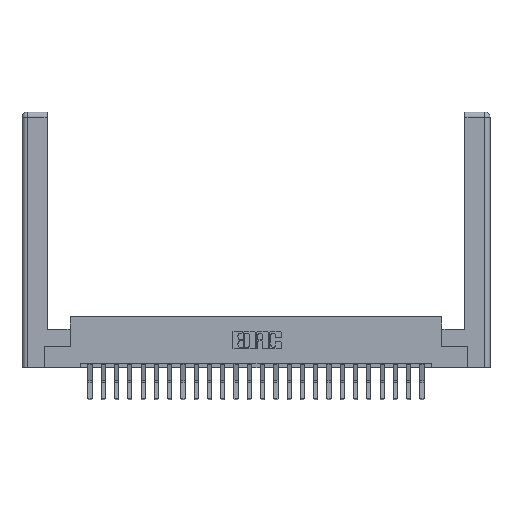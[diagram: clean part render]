
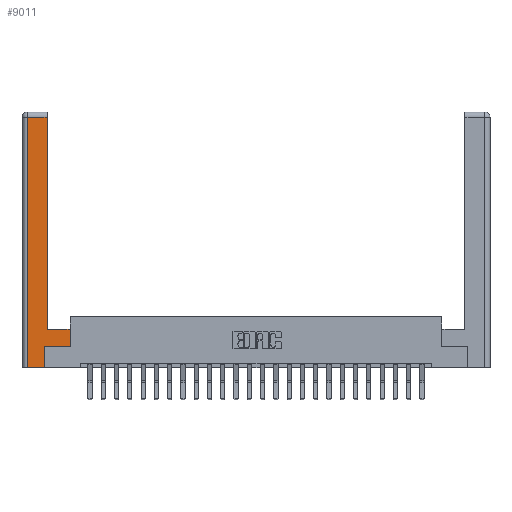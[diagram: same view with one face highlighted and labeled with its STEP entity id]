
A CAD part, top view. The second image highlights one B-rep face of the part: STEP entity #9011.
In plain terms, the highlighted planar face has unit normal (0, 0, 1).
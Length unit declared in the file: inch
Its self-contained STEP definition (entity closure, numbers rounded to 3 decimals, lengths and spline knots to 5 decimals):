
#345 = DIRECTION ( 'NONE',  ( 0., -1., 0. ) ) ;
#403 = FACE_OUTER_BOUND ( 'NONE', #6809, .T. ) ;
#785 = EDGE_CURVE ( 'NONE', #9974, #18784, #2170, .T. ) ;
#1206 = VECTOR ( 'NONE', #19770, 39.37008 ) ;
#2170 = LINE ( 'NONE', #8299, #19724 ) ;
#2855 = CARTESIAN_POINT ( 'NONE',  ( 0.295, 0.45, 0. ) ) ;
#3918 = ORIENTED_EDGE ( 'NONE', *, *, #5285, .T. ) ;
#4222 = ORIENTED_EDGE ( 'NONE', *, *, #16011, .T. ) ;
#4379 = CARTESIAN_POINT ( 'NONE',  ( 0.565, 0.45, 0. ) ) ;
#4415 = CARTESIAN_POINT ( 'NONE',  ( 0.265, 0.245, 0. ) ) ;
#4665 = VECTOR ( 'NONE', #4693, 39.37008 ) ;
#4693 = DIRECTION ( 'NONE',  ( 1., 0., 0. ) ) ;
#5285 = EDGE_CURVE ( 'NONE', #18784, #9771, #23835, .T. ) ;
#6759 = LINE ( 'NONE', #23803, #4665 ) ;
#6809 = EDGE_LOOP ( 'NONE', ( #21625, #19039, #19291, #3918, #19736, #19445, #9357, #4222 ) ) ;
#7153 = DIRECTION ( 'NONE',  ( 0., 0., -1. ) ) ;
#8011 = EDGE_CURVE ( 'NONE', #9771, #23929, #17389, .T. ) ;
#8299 = CARTESIAN_POINT ( 'NONE',  ( 0.0615, 0., 0. ) ) ;
#8806 = DIRECTION ( 'NONE',  ( -1., 0., 0. ) ) ;
#8950 = VECTOR ( 'NONE', #11927, 39.37008 ) ;
#8970 = VECTOR ( 'NONE', #15876, 39.37008 ) ;
#9011 = ADVANCED_FACE ( 'NONE', ( #403 ), #10373, .F. ) ;
#9092 = EDGE_CURVE ( 'NONE', #23929, #13352, #6759, .T. ) ;
#9189 = EDGE_CURVE ( 'NONE', #24588, #10053, #17122, .T. ) ;
#9357 = ORIENTED_EDGE ( 'NONE', *, *, #20486, .T. ) ;
#9771 = VERTEX_POINT ( 'NONE', #15657 ) ;
#9974 = VERTEX_POINT ( 'NONE', #13013 ) ;
#10053 = VERTEX_POINT ( 'NONE', #19138 ) ;
#10373 = PLANE ( 'NONE',  #14374 ) ;
#11901 = LINE ( 'NONE', #4379, #21228 ) ;
#11927 = DIRECTION ( 'NONE',  ( 0., 1., 0. ) ) ;
#11974 = CARTESIAN_POINT ( 'NONE',  ( 0.295, 3., 0. ) ) ;
#12408 = LINE ( 'NONE', #19405, #12727 ) ;
#12562 = CARTESIAN_POINT ( 'NONE',  ( 0., 0., 0. ) ) ;
#12727 = VECTOR ( 'NONE', #15801, 39.37008 ) ;
#12949 = CARTESIAN_POINT ( 'NONE',  ( 0.565, 0.245, 0. ) ) ;
#13013 = CARTESIAN_POINT ( 'NONE',  ( 0.0615, 2.94, 0. ) ) ;
#13352 = VERTEX_POINT ( 'NONE', #12949 ) ;
#13802 = CARTESIAN_POINT ( 'NONE',  ( 0.265, 0.245, 0. ) ) ;
#14374 = AXIS2_PLACEMENT_3D ( 'NONE', #12562, #7153, #14779 ) ;
#14396 = CARTESIAN_POINT ( 'NONE',  ( 0.565, 0.45, 0. ) ) ;
#14779 = DIRECTION ( 'NONE',  ( -1., 0., 0. ) ) ;
#14842 = CARTESIAN_POINT ( 'NONE',  ( 0.295, 0.45, 0. ) ) ;
#15657 = CARTESIAN_POINT ( 'NONE',  ( 0.265, 0., 0. ) ) ;
#15801 = DIRECTION ( 'NONE',  ( -1., 0., 0. ) ) ;
#15874 = CARTESIAN_POINT ( 'NONE',  ( 0.0615, 0., 0. ) ) ;
#15876 = DIRECTION ( 'NONE',  ( 0., 1., 0. ) ) ;
#16011 = EDGE_CURVE ( 'NONE', #19501, #24588, #24193, .T. ) ;
#16039 = DIRECTION ( 'NONE',  ( 0., 1., 0. ) ) ;
#16360 = EDGE_CURVE ( 'NONE', #10053, #9974, #12408, .T. ) ;
#16387 = VECTOR ( 'NONE', #8806, 39.37008 ) ;
#17122 = LINE ( 'NONE', #11974, #8970 ) ;
#17367 = CARTESIAN_POINT ( 'NONE',  ( 0.265, 0., 0. ) ) ;
#17389 = LINE ( 'NONE', #13802, #8950 ) ;
#18784 = VERTEX_POINT ( 'NONE', #15874 ) ;
#19039 = ORIENTED_EDGE ( 'NONE', *, *, #16360, .T. ) ;
#19138 = CARTESIAN_POINT ( 'NONE',  ( 0.295, 2.94, 0. ) ) ;
#19291 = ORIENTED_EDGE ( 'NONE', *, *, #785, .T. ) ;
#19405 = CARTESIAN_POINT ( 'NONE',  ( 0.0615, 2.94, 0. ) ) ;
#19445 = ORIENTED_EDGE ( 'NONE', *, *, #9092, .T. ) ;
#19501 = VERTEX_POINT ( 'NONE', #14396 ) ;
#19724 = VECTOR ( 'NONE', #345, 39.37008 ) ;
#19736 = ORIENTED_EDGE ( 'NONE', *, *, #8011, .T. ) ;
#19770 = DIRECTION ( 'NONE',  ( 1., 0., 0. ) ) ;
#20486 = EDGE_CURVE ( 'NONE', #13352, #19501, #11901, .T. ) ;
#21228 = VECTOR ( 'NONE', #16039, 39.37008 ) ;
#21625 = ORIENTED_EDGE ( 'NONE', *, *, #9189, .T. ) ;
#23803 = CARTESIAN_POINT ( 'NONE',  ( 0.565, 0.245, 0. ) ) ;
#23835 = LINE ( 'NONE', #17367, #1206 ) ;
#23929 = VERTEX_POINT ( 'NONE', #4415 ) ;
#24193 = LINE ( 'NONE', #2855, #16387 ) ;
#24588 = VERTEX_POINT ( 'NONE', #14842 ) ;
